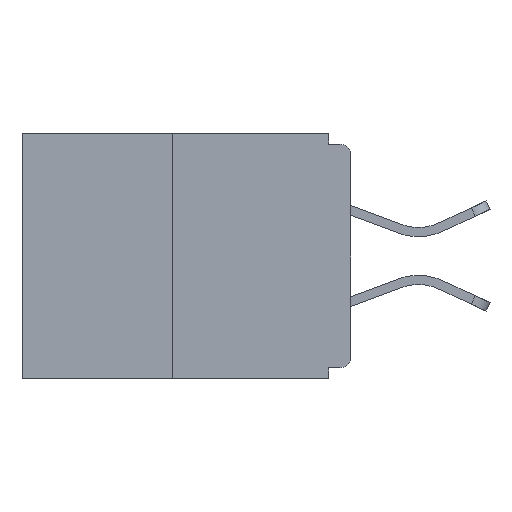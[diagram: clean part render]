
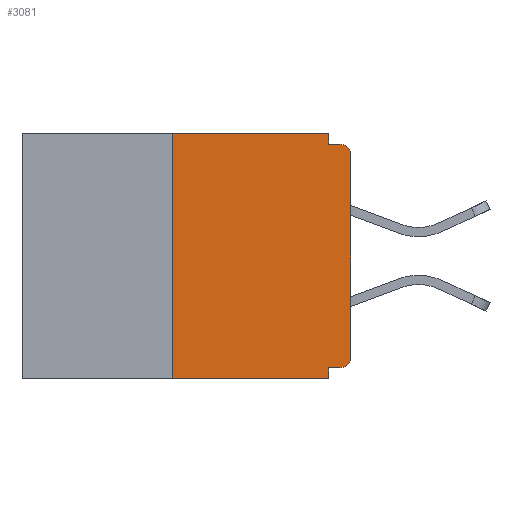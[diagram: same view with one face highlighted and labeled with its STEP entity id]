
A CAD part, left-side view. The second image highlights one B-rep face of the part: STEP entity #3081.
In plain terms, the highlighted planar face has unit normal (-1, 0, 0).
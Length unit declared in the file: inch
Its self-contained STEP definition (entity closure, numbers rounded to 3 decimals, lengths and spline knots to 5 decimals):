
#21 = DIRECTION ( 'NONE',  ( 0., 0., -1. ) ) ;
#23 = CARTESIAN_POINT ( 'NONE',  ( 0., 0., -0.03 ) ) ;
#132 = ORIENTED_EDGE ( 'NONE', *, *, #13348, .F. ) ;
#137 = AXIS2_PLACEMENT_3D ( 'NONE', #2478, #6022, #3513 ) ;
#186 = LINE ( 'NONE', #12672, #2949 ) ;
#273 = CARTESIAN_POINT ( 'NONE',  ( 0., 0.015, -0.328 ) ) ;
#358 = LINE ( 'NONE', #1996, #3124 ) ;
#435 = CARTESIAN_POINT ( 'NONE',  ( 0., 0., -0.313 ) ) ;
#484 = EDGE_CURVE ( 'NONE', #9447, #9228, #14687, .T. ) ;
#781 = AXIS2_PLACEMENT_3D ( 'NONE', #9161, #9400, #21 ) ;
#850 = ORIENTED_EDGE ( 'NONE', *, *, #904, .T. ) ;
#904 = EDGE_CURVE ( 'NONE', #9303, #9447, #7892, .T. ) ;
#1430 = ORIENTED_EDGE ( 'NONE', *, *, #6493, .T. ) ;
#1560 = LINE ( 'NONE', #4600, #3598 ) ;
#1696 = EDGE_LOOP ( 'NONE', ( #132, #11032, #1430, #8766, #4320, #850, #5338, #2284, #7400, #6658 ) ) ;
#1776 = DIRECTION ( 'NONE',  ( 0., -1., 0. ) ) ;
#1845 = VERTEX_POINT ( 'NONE', #5563 ) ;
#1873 = VECTOR ( 'NONE', #5717, 39.37008 ) ;
#1996 = CARTESIAN_POINT ( 'NONE',  ( 0., 0.031, 0. ) ) ;
#2137 = CARTESIAN_POINT ( 'NONE',  ( 0., 0.015, -0.03 ) ) ;
#2284 = ORIENTED_EDGE ( 'NONE', *, *, #12857, .T. ) ;
#2478 = CARTESIAN_POINT ( 'NONE',  ( 0., 0.46, 0. ) ) ;
#2587 = CARTESIAN_POINT ( 'NONE',  ( 0., 0.031, -0.343 ) ) ;
#2656 = LINE ( 'NONE', #11092, #3594 ) ;
#2724 = CARTESIAN_POINT ( 'NONE',  ( 0., 0.031, -0.015 ) ) ;
#2949 = VECTOR ( 'NONE', #5698, 39.37008 ) ;
#3081 = ADVANCED_FACE ( 'NONE', ( #13865 ), #10550, .F. ) ;
#3124 = VECTOR ( 'NONE', #3229, 39.37008 ) ;
#3162 = VERTEX_POINT ( 'NONE', #2724 ) ;
#3229 = DIRECTION ( 'NONE',  ( 0., 0., -1. ) ) ;
#3287 = DIRECTION ( 'NONE',  ( -1., 0., 0. ) ) ;
#3513 = DIRECTION ( 'NONE',  ( 0., 0., -1. ) ) ;
#3594 = VECTOR ( 'NONE', #12117, 39.37008 ) ;
#3598 = VECTOR ( 'NONE', #10499, 39.37008 ) ;
#3749 = LINE ( 'NONE', #11129, #4662 ) ;
#3933 = DIRECTION ( 'NONE',  ( 0., -1., 0. ) ) ;
#4320 = ORIENTED_EDGE ( 'NONE', *, *, #6615, .F. ) ;
#4576 = DIRECTION ( 'NONE',  ( 0., 0., -1. ) ) ;
#4600 = CARTESIAN_POINT ( 'NONE',  ( 0., 0.25, 0. ) ) ;
#4662 = VECTOR ( 'NONE', #1776, 39.37008 ) ;
#4885 = AXIS2_PLACEMENT_3D ( 'NONE', #2137, #3287, #4576 ) ;
#5338 = ORIENTED_EDGE ( 'NONE', *, *, #484, .T. ) ;
#5563 = CARTESIAN_POINT ( 'NONE',  ( 0., 0.25, 0. ) ) ;
#5698 = DIRECTION ( 'NONE',  ( 0., 0., -1. ) ) ;
#5717 = DIRECTION ( 'NONE',  ( 0., 0., 1. ) ) ;
#5965 = CIRCLE ( 'NONE', #4885, 0.015 ) ;
#6022 = DIRECTION ( 'NONE',  ( 1., 0., 0. ) ) ;
#6282 = VECTOR ( 'NONE', #3933, 39.37008 ) ;
#6493 = EDGE_CURVE ( 'NONE', #12456, #7700, #12900, .T. ) ;
#6615 = EDGE_CURVE ( 'NONE', #9303, #14555, #2656, .T. ) ;
#6658 = ORIENTED_EDGE ( 'NONE', *, *, #9012, .F. ) ;
#7400 = ORIENTED_EDGE ( 'NONE', *, *, #13938, .F. ) ;
#7700 = VERTEX_POINT ( 'NONE', #2587 ) ;
#7892 = CIRCLE ( 'NONE', #781, 0.015 ) ;
#8287 = LINE ( 'NONE', #9679, #6282 ) ;
#8352 = CARTESIAN_POINT ( 'NONE',  ( 0., 0.46, -0.343 ) ) ;
#8766 = ORIENTED_EDGE ( 'NONE', *, *, #9072, .F. ) ;
#9012 = EDGE_CURVE ( 'NONE', #12327, #3162, #358, .T. ) ;
#9072 = EDGE_CURVE ( 'NONE', #14555, #7700, #186, .T. ) ;
#9161 = CARTESIAN_POINT ( 'NONE',  ( 0., 0.015, -0.313 ) ) ;
#9228 = VERTEX_POINT ( 'NONE', #23 ) ;
#9269 = CARTESIAN_POINT ( 'NONE',  ( 0., 0.25, -0.343 ) ) ;
#9303 = VERTEX_POINT ( 'NONE', #273 ) ;
#9400 = DIRECTION ( 'NONE',  ( -1., 0., 0. ) ) ;
#9447 = VERTEX_POINT ( 'NONE', #435 ) ;
#9679 = CARTESIAN_POINT ( 'NONE',  ( 0., 0., -0.015 ) ) ;
#10499 = DIRECTION ( 'NONE',  ( 0., 0., 1. ) ) ;
#10550 = PLANE ( 'NONE',  #137 ) ;
#10755 = VECTOR ( 'NONE', #13037, 39.37008 ) ;
#11032 = ORIENTED_EDGE ( 'NONE', *, *, #11853, .F. ) ;
#11092 = CARTESIAN_POINT ( 'NONE',  ( 0., 0., -0.328 ) ) ;
#11129 = CARTESIAN_POINT ( 'NONE',  ( 0., 0.46, 0. ) ) ;
#11358 = CARTESIAN_POINT ( 'NONE',  ( 0., 0.031, 0. ) ) ;
#11853 = EDGE_CURVE ( 'NONE', #12456, #1845, #1560, .T. ) ;
#12117 = DIRECTION ( 'NONE',  ( 0., 1., 0. ) ) ;
#12327 = VERTEX_POINT ( 'NONE', #11358 ) ;
#12456 = VERTEX_POINT ( 'NONE', #9269 ) ;
#12672 = CARTESIAN_POINT ( 'NONE',  ( 0., 0.031, -0.343 ) ) ;
#12857 = EDGE_CURVE ( 'NONE', #9228, #13019, #5965, .T. ) ;
#12900 = LINE ( 'NONE', #8352, #10755 ) ;
#12978 = CARTESIAN_POINT ( 'NONE',  ( 0., 0.015, -0.015 ) ) ;
#13019 = VERTEX_POINT ( 'NONE', #12978 ) ;
#13037 = DIRECTION ( 'NONE',  ( 0., -1., 0. ) ) ;
#13348 = EDGE_CURVE ( 'NONE', #1845, #12327, #3749, .T. ) ;
#13539 = CARTESIAN_POINT ( 'NONE',  ( 0., 0.031, -0.328 ) ) ;
#13833 = CARTESIAN_POINT ( 'NONE',  ( 0., 0., 0. ) ) ;
#13865 = FACE_OUTER_BOUND ( 'NONE', #1696, .T. ) ;
#13938 = EDGE_CURVE ( 'NONE', #3162, #13019, #8287, .T. ) ;
#14555 = VERTEX_POINT ( 'NONE', #13539 ) ;
#14687 = LINE ( 'NONE', #13833, #1873 ) ;
